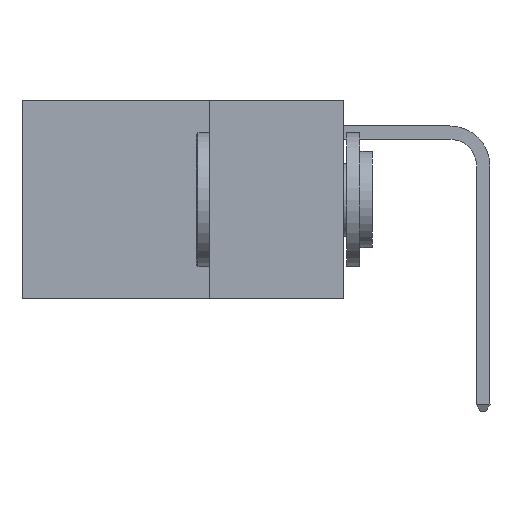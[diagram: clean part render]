
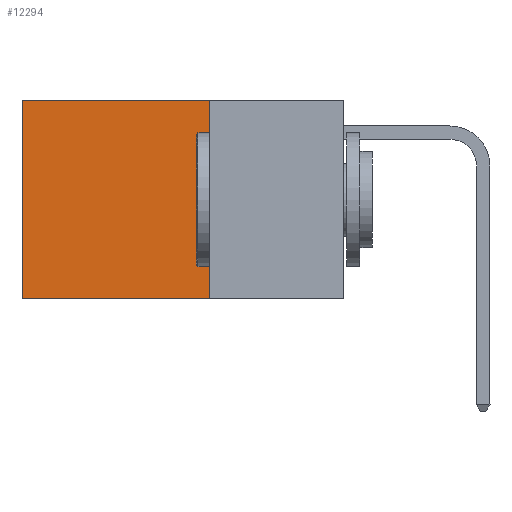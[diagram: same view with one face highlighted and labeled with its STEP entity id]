
A CAD part, left-side view. The second image highlights one B-rep face of the part: STEP entity #12294.
In plain terms, the highlighted planar face has unit normal (-1, 0, 0).
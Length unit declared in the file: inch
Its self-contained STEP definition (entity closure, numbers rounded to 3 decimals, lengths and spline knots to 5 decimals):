
#1006 = LINE ( 'NONE', #4419, #8603 ) ;
#1195 = VECTOR ( 'NONE', #8576, 39.37008 ) ;
#1322 = DIRECTION ( 'NONE',  ( 0., 0., -1. ) ) ;
#1796 = VERTEX_POINT ( 'NONE', #13420 ) ;
#1819 = VECTOR ( 'NONE', #7915, 39.37008 ) ;
#2736 = AXIS2_PLACEMENT_3D ( 'NONE', #2935, #13300, #4464 ) ;
#2935 = CARTESIAN_POINT ( 'NONE',  ( 0.2625, 0.25, 0. ) ) ;
#3239 = VERTEX_POINT ( 'NONE', #17348 ) ;
#3938 = EDGE_CURVE ( 'NONE', #12956, #1796, #18369, .T. ) ;
#4419 = CARTESIAN_POINT ( 'NONE',  ( 0.2625, 0.6, 0. ) ) ;
#4464 = DIRECTION ( 'NONE',  ( 0., 0., -1. ) ) ;
#4731 = FACE_OUTER_BOUND ( 'NONE', #11096, .T. ) ;
#4939 = EDGE_CURVE ( 'NONE', #3239, #19026, #9824, .T. ) ;
#6406 = VECTOR ( 'NONE', #17429, 39.37008 ) ;
#6575 = EDGE_CURVE ( 'NONE', #1796, #19026, #1006, .T. ) ;
#7105 = CARTESIAN_POINT ( 'NONE',  ( 0.2625, 0.25, 0. ) ) ;
#7666 = ORIENTED_EDGE ( 'NONE', *, *, #3938, .T. ) ;
#7915 = DIRECTION ( 'NONE',  ( 0., 1., 0. ) ) ;
#8020 = CARTESIAN_POINT ( 'NONE',  ( 0.2625, 0.25, -0.37 ) ) ;
#8576 = DIRECTION ( 'NONE',  ( 0., 0., -1. ) ) ;
#8603 = VECTOR ( 'NONE', #1322, 39.37008 ) ;
#8780 = LINE ( 'NONE', #7105, #1195 ) ;
#9824 = LINE ( 'NONE', #8020, #1819 ) ;
#9952 = EDGE_CURVE ( 'NONE', #12956, #3239, #8780, .T. ) ;
#10496 = CARTESIAN_POINT ( 'NONE',  ( 0.2625, 0.25, 0. ) ) ;
#11096 = EDGE_LOOP ( 'NONE', ( #17709, #14434, #16068, #7666 ) ) ;
#11841 = PLANE ( 'NONE',  #2736 ) ;
#12294 = ADVANCED_FACE ( 'NONE', ( #4731 ), #11841, .F. ) ;
#12956 = VERTEX_POINT ( 'NONE', #10496 ) ;
#13300 = DIRECTION ( 'NONE',  ( 1., 0., 0. ) ) ;
#13420 = CARTESIAN_POINT ( 'NONE',  ( 0.2625, 0.6, 0. ) ) ;
#14434 = ORIENTED_EDGE ( 'NONE', *, *, #4939, .F. ) ;
#15512 = CARTESIAN_POINT ( 'NONE',  ( 0.2625, 0.6, -0.37 ) ) ;
#16068 = ORIENTED_EDGE ( 'NONE', *, *, #9952, .F. ) ;
#17348 = CARTESIAN_POINT ( 'NONE',  ( 0.2625, 0.25, -0.37 ) ) ;
#17429 = DIRECTION ( 'NONE',  ( 0., 1., 0. ) ) ;
#17471 = CARTESIAN_POINT ( 'NONE',  ( 0.2625, 0.25, 0. ) ) ;
#17709 = ORIENTED_EDGE ( 'NONE', *, *, #6575, .T. ) ;
#18369 = LINE ( 'NONE', #17471, #6406 ) ;
#19026 = VERTEX_POINT ( 'NONE', #15512 ) ;
